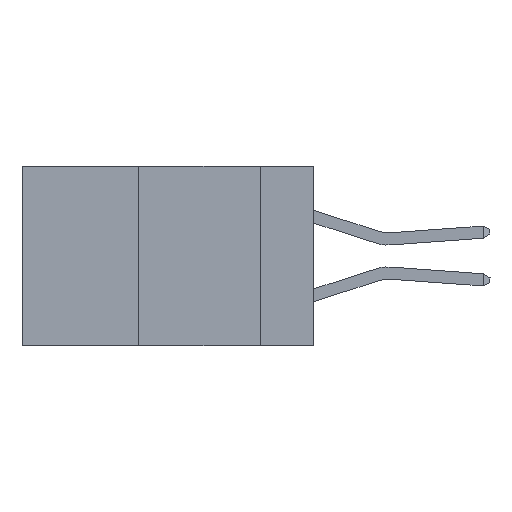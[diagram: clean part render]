
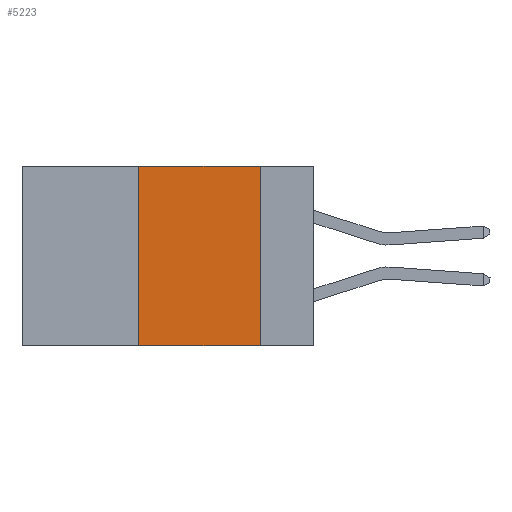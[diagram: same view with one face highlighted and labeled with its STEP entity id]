
A CAD part, left-side view. The second image highlights one B-rep face of the part: STEP entity #5223.
In plain terms, the highlighted planar face has unit normal (-1, 0, 0).
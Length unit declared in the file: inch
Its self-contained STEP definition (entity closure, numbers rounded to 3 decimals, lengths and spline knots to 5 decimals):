
#239 = EDGE_LOOP ( 'NONE', ( #39421, #7383, #26524, #20692 ) ) ;
#1928 = VERTEX_POINT ( 'NONE', #38795 ) ;
#2113 = DIRECTION ( 'NONE',  ( 1., 0., 0. ) ) ;
#5207 = PLANE ( 'NONE',  #20274 ) ;
#5223 = ADVANCED_FACE ( 'NONE', ( #32886 ), #5207, .F. ) ;
#5615 = VECTOR ( 'NONE', #14703, 39.37008 ) ;
#7383 = ORIENTED_EDGE ( 'NONE', *, *, #29326, .F. ) ;
#11585 = LINE ( 'NONE', #27482, #35808 ) ;
#11810 = LINE ( 'NONE', #23596, #5615 ) ;
#14703 = DIRECTION ( 'NONE',  ( 0., -1., 0. ) ) ;
#14704 = DIRECTION ( 'NONE',  ( 0., 0., -1. ) ) ;
#15670 = CARTESIAN_POINT ( 'NONE',  ( 0., 0.11, 0. ) ) ;
#16089 = LINE ( 'NONE', #15670, #30184 ) ;
#17791 = CARTESIAN_POINT ( 'NONE',  ( 0., 0.6, 0. ) ) ;
#20274 = AXIS2_PLACEMENT_3D ( 'NONE', #17791, #2113, #14704 ) ;
#20692 = ORIENTED_EDGE ( 'NONE', *, *, #24820, .T. ) ;
#23596 = CARTESIAN_POINT ( 'NONE',  ( 0., 0.6, 0. ) ) ;
#23660 = CARTESIAN_POINT ( 'NONE',  ( 0., 0.36, 0. ) ) ;
#24175 = DIRECTION ( 'NONE',  ( 0., -1., 0. ) ) ;
#24615 = CARTESIAN_POINT ( 'NONE',  ( 0., 0.36, 0. ) ) ;
#24820 = EDGE_CURVE ( 'NONE', #32047, #25960, #11585, .T. ) ;
#25960 = VERTEX_POINT ( 'NONE', #37693 ) ;
#26524 = ORIENTED_EDGE ( 'NONE', *, *, #38587, .F. ) ;
#27482 = CARTESIAN_POINT ( 'NONE',  ( 0., 0.6, -0.37 ) ) ;
#28083 = VERTEX_POINT ( 'NONE', #24615 ) ;
#28275 = DIRECTION ( 'NONE',  ( 0., 0., -1. ) ) ;
#29326 = EDGE_CURVE ( 'NONE', #28083, #1928, #11810, .T. ) ;
#29571 = VECTOR ( 'NONE', #36252, 39.37008 ) ;
#29858 = LINE ( 'NONE', #23660, #29571 ) ;
#30184 = VECTOR ( 'NONE', #28275, 39.37008 ) ;
#32047 = VERTEX_POINT ( 'NONE', #32498 ) ;
#32498 = CARTESIAN_POINT ( 'NONE',  ( 0., 0.36, -0.37 ) ) ;
#32886 = FACE_OUTER_BOUND ( 'NONE', #239, .T. ) ;
#35808 = VECTOR ( 'NONE', #24175, 39.37008 ) ;
#36252 = DIRECTION ( 'NONE',  ( 0., 0., 1. ) ) ;
#36615 = EDGE_CURVE ( 'NONE', #1928, #25960, #16089, .T. ) ;
#37693 = CARTESIAN_POINT ( 'NONE',  ( 0., 0.11, -0.37 ) ) ;
#38587 = EDGE_CURVE ( 'NONE', #32047, #28083, #29858, .T. ) ;
#38795 = CARTESIAN_POINT ( 'NONE',  ( 0., 0.11, 0. ) ) ;
#39421 = ORIENTED_EDGE ( 'NONE', *, *, #36615, .F. ) ;
